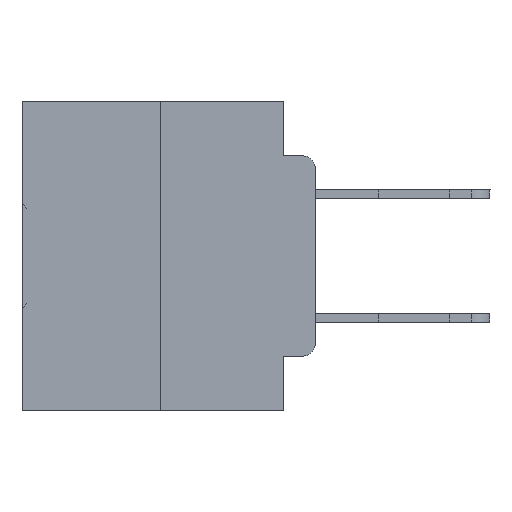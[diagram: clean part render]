
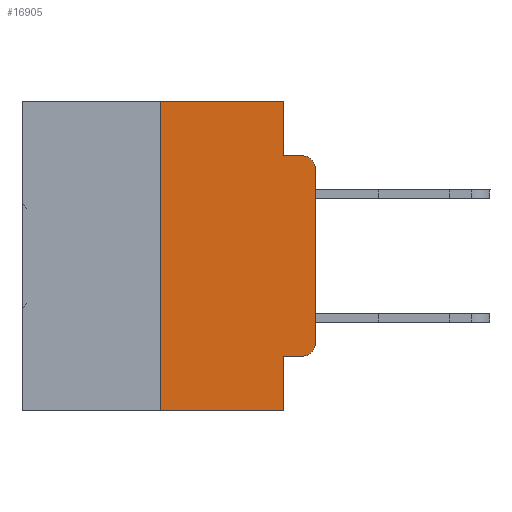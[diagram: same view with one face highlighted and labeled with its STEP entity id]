
A CAD part, left-side view. The second image highlights one B-rep face of the part: STEP entity #16905.
In plain terms, the highlighted planar face has unit normal (-1, 0, 0).
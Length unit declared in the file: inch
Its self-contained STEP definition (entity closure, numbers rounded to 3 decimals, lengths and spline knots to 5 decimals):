
#753 = VERTEX_POINT ( 'NONE', #21222 ) ;
#1548 = EDGE_CURVE ( 'NONE', #24092, #2871, #27299, .T. ) ;
#1615 = DIRECTION ( 'NONE',  ( 0., 0., 1. ) ) ;
#1630 = AXIS2_PLACEMENT_3D ( 'NONE', #12959, #24294, #18447 ) ;
#1882 = ORIENTED_EDGE ( 'NONE', *, *, #33995, .T. ) ;
#1918 = CARTESIAN_POINT ( 'NONE',  ( 0., 0., -0.3915 ) ) ;
#2187 = DIRECTION ( 'NONE',  ( 0., -1., 0. ) ) ;
#2209 = VECTOR ( 'NONE', #1615, 39.37008 ) ;
#2871 = VERTEX_POINT ( 'NONE', #26079 ) ;
#2890 = VECTOR ( 'NONE', #25623, 39.37008 ) ;
#3259 = VECTOR ( 'NONE', #14500, 39.37008 ) ;
#3468 = VECTOR ( 'NONE', #23989, 39.37008 ) ;
#3960 = AXIS2_PLACEMENT_3D ( 'NONE', #8947, #12436, #34587 ) ;
#4182 = VERTEX_POINT ( 'NONE', #13169 ) ;
#4369 = LINE ( 'NONE', #18326, #3468 ) ;
#4808 = CARTESIAN_POINT ( 'NONE',  ( 0., 0.25, -0.5 ) ) ;
#5319 = CARTESIAN_POINT ( 'NONE',  ( 0., 0.25, 0. ) ) ;
#5474 = DIRECTION ( 'NONE',  ( 1., 0., 0. ) ) ;
#6228 = VERTEX_POINT ( 'NONE', #4808 ) ;
#6583 = CARTESIAN_POINT ( 'NONE',  ( 0., 0.473, -0.5 ) ) ;
#6940 = EDGE_CURVE ( 'NONE', #6228, #32165, #8977, .T. ) ;
#7747 = VECTOR ( 'NONE', #32855, 39.37008 ) ;
#8041 = CARTESIAN_POINT ( 'NONE',  ( 0., 0.051, 0. ) ) ;
#8118 = ORIENTED_EDGE ( 'NONE', *, *, #6940, .T. ) ;
#8796 = EDGE_CURVE ( 'NONE', #9025, #13474, #15684, .T. ) ;
#8947 = CARTESIAN_POINT ( 'NONE',  ( 0., 0.02, -0.3915 ) ) ;
#8977 = LINE ( 'NONE', #6583, #3259 ) ;
#9025 = VERTEX_POINT ( 'NONE', #27420 ) ;
#10377 = EDGE_CURVE ( 'NONE', #33791, #2871, #31516, .T. ) ;
#12436 = DIRECTION ( 'NONE',  ( -1., 0., 0. ) ) ;
#12642 = ORIENTED_EDGE ( 'NONE', *, *, #17626, .F. ) ;
#12682 = VERTEX_POINT ( 'NONE', #5319 ) ;
#12959 = CARTESIAN_POINT ( 'NONE',  ( 0., 0.02, -0.1085 ) ) ;
#13150 = EDGE_CURVE ( 'NONE', #4182, #32165, #28700, .T. ) ;
#13169 = CARTESIAN_POINT ( 'NONE',  ( 0., 0.051, -0.4115 ) ) ;
#13474 = VERTEX_POINT ( 'NONE', #1918 ) ;
#13651 = VECTOR ( 'NONE', #2187, 39.37008 ) ;
#14500 = DIRECTION ( 'NONE',  ( 0., -1., 0. ) ) ;
#15103 = EDGE_LOOP ( 'NONE', ( #30483, #21331, #26601, #12642, #18204, #30912, #8118, #18390, #1882, #16371 ) ) ;
#15118 = CARTESIAN_POINT ( 'NONE',  ( 0., 0., -0.1085 ) ) ;
#15420 = CARTESIAN_POINT ( 'NONE',  ( 0., 0.051, -0.0885 ) ) ;
#15571 = CARTESIAN_POINT ( 'NONE',  ( 0., 0., 0. ) ) ;
#15684 = CIRCLE ( 'NONE', #3960, 0.02 ) ;
#16371 = ORIENTED_EDGE ( 'NONE', *, *, #8796, .T. ) ;
#16673 = DIRECTION ( 'NONE',  ( 0., 0., -1. ) ) ;
#16905 = ADVANCED_FACE ( 'NONE', ( #22347 ), #22170, .F. ) ;
#17626 = EDGE_CURVE ( 'NONE', #753, #24092, #35962, .T. ) ;
#18204 = ORIENTED_EDGE ( 'NONE', *, *, #30530, .F. ) ;
#18326 = CARTESIAN_POINT ( 'NONE',  ( 0., 0.25, 0. ) ) ;
#18390 = ORIENTED_EDGE ( 'NONE', *, *, #13150, .F. ) ;
#18447 = DIRECTION ( 'NONE',  ( 0., 0., -1. ) ) ;
#19462 = CARTESIAN_POINT ( 'NONE',  ( 0., 0.051, -0.4115 ) ) ;
#21144 = LINE ( 'NONE', #19462, #21196 ) ;
#21196 = VECTOR ( 'NONE', #27531, 39.37008 ) ;
#21222 = CARTESIAN_POINT ( 'NONE',  ( 0., 0.051, 0. ) ) ;
#21331 = ORIENTED_EDGE ( 'NONE', *, *, #10377, .T. ) ;
#21494 = CARTESIAN_POINT ( 'NONE',  ( 0., 0.051, 0. ) ) ;
#22170 = PLANE ( 'NONE',  #25856 ) ;
#22347 = FACE_OUTER_BOUND ( 'NONE', #15103, .T. ) ;
#23989 = DIRECTION ( 'NONE',  ( 0., 0., 1. ) ) ;
#24022 = VECTOR ( 'NONE', #30424, 39.37008 ) ;
#24092 = VERTEX_POINT ( 'NONE', #32041 ) ;
#24294 = DIRECTION ( 'NONE',  ( -1., 0., 0. ) ) ;
#25623 = DIRECTION ( 'NONE',  ( 0., -1., 0. ) ) ;
#25803 = LINE ( 'NONE', #33872, #2890 ) ;
#25856 = AXIS2_PLACEMENT_3D ( 'NONE', #33350, #5474, #16673 ) ;
#26079 = CARTESIAN_POINT ( 'NONE',  ( 0., 0.02, -0.0885 ) ) ;
#26193 = LINE ( 'NONE', #15571, #2209 ) ;
#26601 = ORIENTED_EDGE ( 'NONE', *, *, #1548, .F. ) ;
#27299 = LINE ( 'NONE', #15420, #13651 ) ;
#27393 = CARTESIAN_POINT ( 'NONE',  ( 0., 0.051, -0.5 ) ) ;
#27420 = CARTESIAN_POINT ( 'NONE',  ( 0., 0.02, -0.4115 ) ) ;
#27531 = DIRECTION ( 'NONE',  ( 0., -1., 0. ) ) ;
#28700 = LINE ( 'NONE', #8041, #24022 ) ;
#28793 = EDGE_CURVE ( 'NONE', #13474, #33791, #26193, .T. ) ;
#30147 = EDGE_CURVE ( 'NONE', #6228, #12682, #4369, .T. ) ;
#30424 = DIRECTION ( 'NONE',  ( 0., 0., -1. ) ) ;
#30483 = ORIENTED_EDGE ( 'NONE', *, *, #28793, .T. ) ;
#30530 = EDGE_CURVE ( 'NONE', #12682, #753, #25803, .T. ) ;
#30912 = ORIENTED_EDGE ( 'NONE', *, *, #30147, .F. ) ;
#31516 = CIRCLE ( 'NONE', #1630, 0.02 ) ;
#32041 = CARTESIAN_POINT ( 'NONE',  ( 0., 0.051, -0.0885 ) ) ;
#32165 = VERTEX_POINT ( 'NONE', #27393 ) ;
#32855 = DIRECTION ( 'NONE',  ( 0., 0., -1. ) ) ;
#33350 = CARTESIAN_POINT ( 'NONE',  ( 0., 0.473, 0. ) ) ;
#33791 = VERTEX_POINT ( 'NONE', #15118 ) ;
#33872 = CARTESIAN_POINT ( 'NONE',  ( 0., 0.473, 0. ) ) ;
#33995 = EDGE_CURVE ( 'NONE', #4182, #9025, #21144, .T. ) ;
#34587 = DIRECTION ( 'NONE',  ( 0., 0., -1. ) ) ;
#35962 = LINE ( 'NONE', #21494, #7747 ) ;
